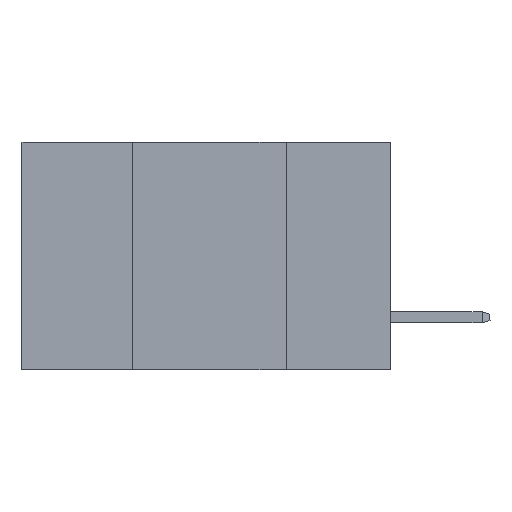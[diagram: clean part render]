
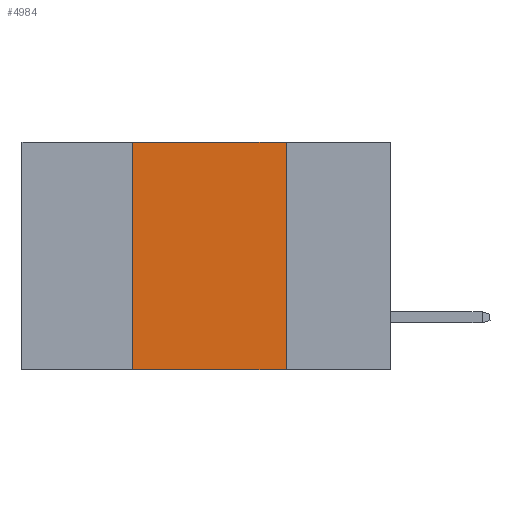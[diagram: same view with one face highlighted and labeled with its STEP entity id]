
A CAD part, left-side view. The second image highlights one B-rep face of the part: STEP entity #4984.
In plain terms, the highlighted planar face has unit normal (-1, 0, 0).
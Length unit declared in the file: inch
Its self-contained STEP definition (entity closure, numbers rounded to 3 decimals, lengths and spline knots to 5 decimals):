
#753 = DIRECTION ( 'NONE',  ( 0., 0., -1. ) ) ;
#800 = DIRECTION ( 'NONE',  ( 0., -1., 0. ) ) ;
#876 = EDGE_CURVE ( 'NONE', #15821, #23963, #6526, .T. ) ;
#1752 = EDGE_CURVE ( 'NONE', #9969, #15119, #12212, .T. ) ;
#1833 = EDGE_CURVE ( 'NONE', #9969, #23963, #16199, .T. ) ;
#3189 = CARTESIAN_POINT ( 'NONE',  ( 0., 0.6, -0.37 ) ) ;
#4984 = ADVANCED_FACE ( 'NONE', ( #8299 ), #9587, .F. ) ;
#5627 = CARTESIAN_POINT ( 'NONE',  ( 0., 0.42, 0. ) ) ;
#5840 = CARTESIAN_POINT ( 'NONE',  ( 0., 0.17, -0.37 ) ) ;
#5957 = ORIENTED_EDGE ( 'NONE', *, *, #876, .F. ) ;
#6156 = ORIENTED_EDGE ( 'NONE', *, *, #8394, .F. ) ;
#6526 = LINE ( 'NONE', #8629, #11919 ) ;
#6836 = VECTOR ( 'NONE', #10104, 39.37008 ) ;
#6883 = DIRECTION ( 'NONE',  ( 0., 0., -1. ) ) ;
#7032 = DIRECTION ( 'NONE',  ( 1., 0., 0. ) ) ;
#7275 = CARTESIAN_POINT ( 'NONE',  ( 0., 0.6, 0. ) ) ;
#7960 = CARTESIAN_POINT ( 'NONE',  ( 0., 0.42, 0. ) ) ;
#8299 = FACE_OUTER_BOUND ( 'NONE', #20379, .T. ) ;
#8394 = EDGE_CURVE ( 'NONE', #15119, #15821, #16871, .T. ) ;
#8629 = CARTESIAN_POINT ( 'NONE',  ( 0., 0.17, 0. ) ) ;
#9587 = PLANE ( 'NONE',  #23944 ) ;
#9969 = VERTEX_POINT ( 'NONE', #13108 ) ;
#10104 = DIRECTION ( 'NONE',  ( 0., 0., 1. ) ) ;
#10280 = ORIENTED_EDGE ( 'NONE', *, *, #1752, .F. ) ;
#11919 = VECTOR ( 'NONE', #753, 39.37008 ) ;
#12212 = LINE ( 'NONE', #7960, #6836 ) ;
#13108 = CARTESIAN_POINT ( 'NONE',  ( 0., 0.42, -0.37 ) ) ;
#15119 = VERTEX_POINT ( 'NONE', #5627 ) ;
#15821 = VERTEX_POINT ( 'NONE', #23788 ) ;
#16199 = LINE ( 'NONE', #3189, #20744 ) ;
#16871 = LINE ( 'NONE', #23700, #21951 ) ;
#20379 = EDGE_LOOP ( 'NONE', ( #5957, #6156, #10280, #21288 ) ) ;
#20744 = VECTOR ( 'NONE', #800, 39.37008 ) ;
#21288 = ORIENTED_EDGE ( 'NONE', *, *, #1833, .T. ) ;
#21951 = VECTOR ( 'NONE', #25586, 39.37008 ) ;
#23700 = CARTESIAN_POINT ( 'NONE',  ( 0., 0.6, 0. ) ) ;
#23788 = CARTESIAN_POINT ( 'NONE',  ( 0., 0.17, 0. ) ) ;
#23944 = AXIS2_PLACEMENT_3D ( 'NONE', #7275, #7032, #6883 ) ;
#23963 = VERTEX_POINT ( 'NONE', #5840 ) ;
#25586 = DIRECTION ( 'NONE',  ( 0., -1., 0. ) ) ;
